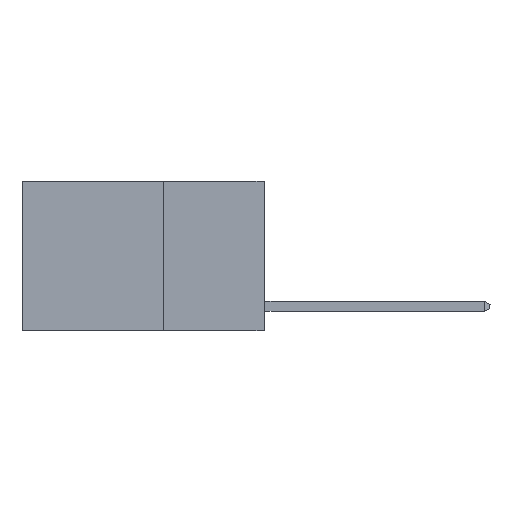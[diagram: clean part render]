
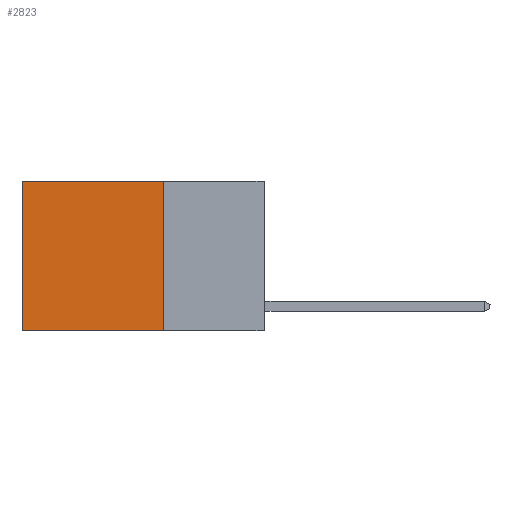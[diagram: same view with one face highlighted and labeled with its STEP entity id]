
A CAD part, left-side view. The second image highlights one B-rep face of the part: STEP entity #2823.
In plain terms, the highlighted planar face has unit normal (-1, 0, 0).
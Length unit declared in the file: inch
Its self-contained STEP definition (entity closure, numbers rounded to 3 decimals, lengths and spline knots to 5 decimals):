
#449 = VECTOR ( 'NONE', #5737, 39.37008 ) ;
#465 = VERTEX_POINT ( 'NONE', #7842 ) ;
#963 = DIRECTION ( 'NONE',  ( 0., 0., -1. ) ) ;
#1895 = VERTEX_POINT ( 'NONE', #8487 ) ;
#2467 = FACE_OUTER_BOUND ( 'NONE', #2611, .T. ) ;
#2514 = ORIENTED_EDGE ( 'NONE', *, *, #10211, .F. ) ;
#2611 = EDGE_LOOP ( 'NONE', ( #11932, #9943, #2514, #6894 ) ) ;
#2823 = ADVANCED_FACE ( 'NONE', ( #2467 ), #5953, .F. ) ;
#2872 = EDGE_CURVE ( 'NONE', #465, #4544, #11944, .T. ) ;
#2942 = CARTESIAN_POINT ( 'NONE',  ( 0.2625, 0.25, 0. ) ) ;
#3056 = DIRECTION ( 'NONE',  ( 0., 1., 0. ) ) ;
#4544 = VERTEX_POINT ( 'NONE', #4646 ) ;
#4646 = CARTESIAN_POINT ( 'NONE',  ( 0.2625, 0.6, 0. ) ) ;
#4951 = LINE ( 'NONE', #9796, #9842 ) ;
#5737 = DIRECTION ( 'NONE',  ( 0., 1., 0. ) ) ;
#5953 = PLANE ( 'NONE',  #8548 ) ;
#6340 = CARTESIAN_POINT ( 'NONE',  ( 0.2625, 0.25, -0.37 ) ) ;
#6747 = CARTESIAN_POINT ( 'NONE',  ( 0.2625, 0.25, -0.37 ) ) ;
#6894 = ORIENTED_EDGE ( 'NONE', *, *, #2872, .T. ) ;
#6924 = DIRECTION ( 'NONE',  ( 1., 0., 0. ) ) ;
#7059 = EDGE_CURVE ( 'NONE', #4544, #1895, #4951, .T. ) ;
#7842 = CARTESIAN_POINT ( 'NONE',  ( 0.2625, 0.25, 0. ) ) ;
#8487 = CARTESIAN_POINT ( 'NONE',  ( 0.2625, 0.6, -0.37 ) ) ;
#8548 = AXIS2_PLACEMENT_3D ( 'NONE', #12647, #6924, #963 ) ;
#8881 = DIRECTION ( 'NONE',  ( 0., 0., -1. ) ) ;
#9188 = VERTEX_POINT ( 'NONE', #6340 ) ;
#9414 = VECTOR ( 'NONE', #3056, 39.37008 ) ;
#9614 = VECTOR ( 'NONE', #8881, 39.37008 ) ;
#9796 = CARTESIAN_POINT ( 'NONE',  ( 0.2625, 0.6, 0. ) ) ;
#9842 = VECTOR ( 'NONE', #10774, 39.37008 ) ;
#9897 = CARTESIAN_POINT ( 'NONE',  ( 0.2625, 0.25, 0. ) ) ;
#9943 = ORIENTED_EDGE ( 'NONE', *, *, #10815, .F. ) ;
#10211 = EDGE_CURVE ( 'NONE', #465, #9188, #12141, .T. ) ;
#10774 = DIRECTION ( 'NONE',  ( 0., 0., -1. ) ) ;
#10815 = EDGE_CURVE ( 'NONE', #9188, #1895, #11248, .T. ) ;
#11248 = LINE ( 'NONE', #6747, #449 ) ;
#11932 = ORIENTED_EDGE ( 'NONE', *, *, #7059, .T. ) ;
#11944 = LINE ( 'NONE', #9897, #9414 ) ;
#12141 = LINE ( 'NONE', #2942, #9614 ) ;
#12647 = CARTESIAN_POINT ( 'NONE',  ( 0.2625, 0.25, 0. ) ) ;
